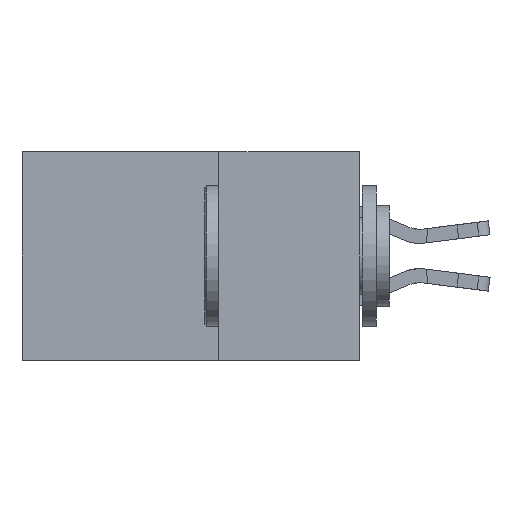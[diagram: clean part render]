
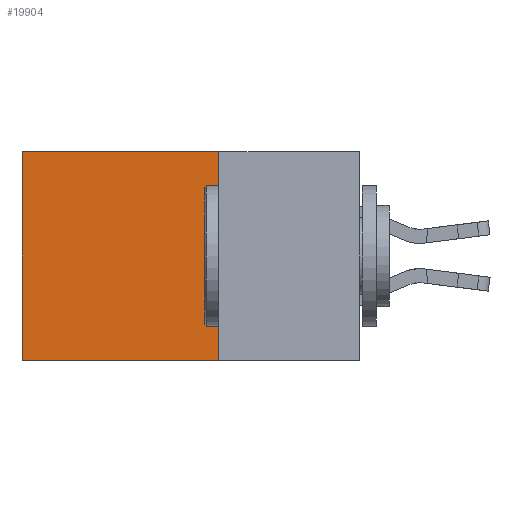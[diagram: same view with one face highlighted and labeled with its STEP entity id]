
A CAD part, left-side view. The second image highlights one B-rep face of the part: STEP entity #19904.
In plain terms, the highlighted planar face has unit normal (-1, 0, 0).
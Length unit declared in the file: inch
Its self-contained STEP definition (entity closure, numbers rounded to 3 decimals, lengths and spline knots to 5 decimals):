
#71 = DIRECTION ( 'NONE',  ( 1., 0., 0. ) ) ;
#1164 = DIRECTION ( 'NONE',  ( 0., 1., 0. ) ) ;
#3010 = CARTESIAN_POINT ( 'NONE',  ( 0.2875, 0.25, 0. ) ) ;
#3183 = VERTEX_POINT ( 'NONE', #25085 ) ;
#3221 = CARTESIAN_POINT ( 'NONE',  ( 0.2875, 0.25, 0. ) ) ;
#3461 = LINE ( 'NONE', #17101, #18149 ) ;
#3704 = DIRECTION ( 'NONE',  ( 0., 1., 0. ) ) ;
#4212 = EDGE_CURVE ( 'NONE', #3183, #33688, #9494, .T. ) ;
#6463 = CARTESIAN_POINT ( 'NONE',  ( 0.2875, 0.6, 0. ) ) ;
#7640 = EDGE_CURVE ( 'NONE', #22813, #3183, #10443, .T. ) ;
#8207 = VECTOR ( 'NONE', #10900, 39.37008 ) ;
#9494 = LINE ( 'NONE', #6463, #31560 ) ;
#9916 = FACE_OUTER_BOUND ( 'NONE', #27115, .T. ) ;
#10443 = LINE ( 'NONE', #21738, #30472 ) ;
#10900 = DIRECTION ( 'NONE',  ( 0., 0., -1. ) ) ;
#13282 = ORIENTED_EDGE ( 'NONE', *, *, #7640, .T. ) ;
#13391 = CARTESIAN_POINT ( 'NONE',  ( 0.2875, 0.25, -0.37 ) ) ;
#15042 = CARTESIAN_POINT ( 'NONE',  ( 0.2875, 0.6, -0.37 ) ) ;
#16790 = LINE ( 'NONE', #3221, #8207 ) ;
#17101 = CARTESIAN_POINT ( 'NONE',  ( 0.2875, 0.25, -0.37 ) ) ;
#17587 = AXIS2_PLACEMENT_3D ( 'NONE', #26021, #71, #23491 ) ;
#18149 = VECTOR ( 'NONE', #1164, 39.37008 ) ;
#19904 = ADVANCED_FACE ( 'NONE', ( #9916 ), #23708, .F. ) ;
#20778 = EDGE_CURVE ( 'NONE', #22813, #25312, #16790, .T. ) ;
#21738 = CARTESIAN_POINT ( 'NONE',  ( 0.2875, 0.25, 0. ) ) ;
#22813 = VERTEX_POINT ( 'NONE', #3010 ) ;
#23491 = DIRECTION ( 'NONE',  ( 0., 0., -1. ) ) ;
#23708 = PLANE ( 'NONE',  #17587 ) ;
#24725 = ORIENTED_EDGE ( 'NONE', *, *, #29958, .F. ) ;
#25085 = CARTESIAN_POINT ( 'NONE',  ( 0.2875, 0.6, 0. ) ) ;
#25312 = VERTEX_POINT ( 'NONE', #13391 ) ;
#26021 = CARTESIAN_POINT ( 'NONE',  ( 0.2875, 0.25, 0. ) ) ;
#27115 = EDGE_LOOP ( 'NONE', ( #30426, #24725, #28303, #13282 ) ) ;
#28303 = ORIENTED_EDGE ( 'NONE', *, *, #20778, .F. ) ;
#29958 = EDGE_CURVE ( 'NONE', #25312, #33688, #3461, .T. ) ;
#29999 = DIRECTION ( 'NONE',  ( 0., 0., -1. ) ) ;
#30426 = ORIENTED_EDGE ( 'NONE', *, *, #4212, .T. ) ;
#30472 = VECTOR ( 'NONE', #3704, 39.37008 ) ;
#31560 = VECTOR ( 'NONE', #29999, 39.37008 ) ;
#33688 = VERTEX_POINT ( 'NONE', #15042 ) ;
